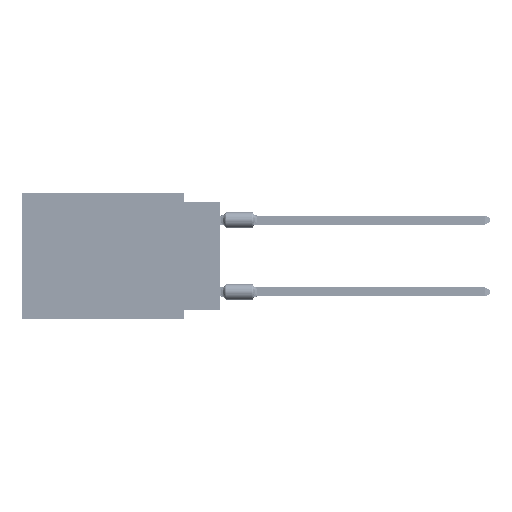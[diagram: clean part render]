
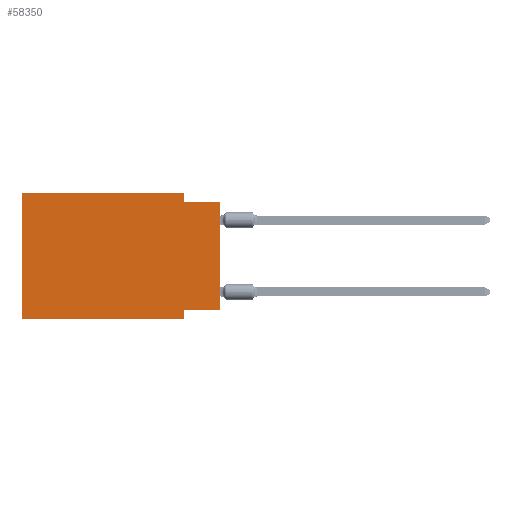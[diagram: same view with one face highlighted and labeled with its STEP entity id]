
A CAD part, left-side view. The second image highlights one B-rep face of the part: STEP entity #58350.
In plain terms, the highlighted planar face has unit normal (-1, 0, 0).
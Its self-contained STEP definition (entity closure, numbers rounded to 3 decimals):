
#297 = DIRECTION ( 'NONE',  ( 0., 0., -1. ) ) ;
#375 = EDGE_CURVE ( 'NONE', #9634, #56281, #20142, .T. ) ;
#571 = VECTOR ( 'NONE', #66476, 1000. ) ;
#1052 = EDGE_CURVE ( 'NONE', #13156, #18423, #66818, .T. ) ;
#1250 = CARTESIAN_POINT ( 'NONE',  ( 0., 0., -8.255 ) ) ;
#3083 = DIRECTION ( 'NONE',  ( 0., -1., 0. ) ) ;
#5361 = DIRECTION ( 'NONE',  ( 1., 0., 0. ) ) ;
#8237 = EDGE_CURVE ( 'NONE', #26276, #27778, #59389, .T. ) ;
#8367 = DIRECTION ( 'NONE',  ( 0., 0., -1. ) ) ;
#9634 = VERTEX_POINT ( 'NONE', #28352 ) ;
#13156 = VERTEX_POINT ( 'NONE', #1250 ) ;
#13600 = CARTESIAN_POINT ( 'NONE',  ( 0., 2.54, 0. ) ) ;
#13890 = DIRECTION ( 'NONE',  ( 0., 0., 1. ) ) ;
#17113 = LINE ( 'NONE', #42981, #43524 ) ;
#18196 = ORIENTED_EDGE ( 'NONE', *, *, #46962, .F. ) ;
#18423 = VERTEX_POINT ( 'NONE', #36624 ) ;
#19375 = DIRECTION ( 'NONE',  ( 0., 1., 0. ) ) ;
#19699 = LINE ( 'NONE', #50859, #60046 ) ;
#20142 = LINE ( 'NONE', #31317, #51988 ) ;
#20844 = ORIENTED_EDGE ( 'NONE', *, *, #36057, .F. ) ;
#22134 = FACE_OUTER_BOUND ( 'NONE', #61054, .T. ) ;
#22450 = CARTESIAN_POINT ( 'NONE',  ( 0., 2.54, 0. ) ) ;
#24410 = VERTEX_POINT ( 'NONE', #68176 ) ;
#25674 = CARTESIAN_POINT ( 'NONE',  ( 0., 2.54, -8.89 ) ) ;
#26276 = VERTEX_POINT ( 'NONE', #50204 ) ;
#27778 = VERTEX_POINT ( 'NONE', #25674 ) ;
#28079 = DIRECTION ( 'NONE',  ( 0., 0., -1. ) ) ;
#28352 = CARTESIAN_POINT ( 'NONE',  ( 0., 13.97, -8.89 ) ) ;
#29003 = VECTOR ( 'NONE', #67531, 1000. ) ;
#30300 = ORIENTED_EDGE ( 'NONE', *, *, #1052, .T. ) ;
#31317 = CARTESIAN_POINT ( 'NONE',  ( 0., 13.97, 0. ) ) ;
#33422 = ORIENTED_EDGE ( 'NONE', *, *, #44740, .F. ) ;
#34199 = LINE ( 'NONE', #62176, #40114 ) ;
#34949 = ORIENTED_EDGE ( 'NONE', *, *, #44660, .T. ) ;
#36057 = EDGE_CURVE ( 'NONE', #46064, #24410, #40180, .T. ) ;
#36302 = ORIENTED_EDGE ( 'NONE', *, *, #42102, .F. ) ;
#36624 = CARTESIAN_POINT ( 'NONE',  ( 0., 0., -0.635 ) ) ;
#37562 = ORIENTED_EDGE ( 'NONE', *, *, #375, .F. ) ;
#39874 = CARTESIAN_POINT ( 'NONE',  ( 0., 0., 0. ) ) ;
#40114 = VECTOR ( 'NONE', #3083, 1000. ) ;
#40180 = LINE ( 'NONE', #13600, #56267 ) ;
#42102 = EDGE_CURVE ( 'NONE', #56281, #46064, #34199, .T. ) ;
#42768 = CARTESIAN_POINT ( 'NONE',  ( 0., 13.97, 0. ) ) ;
#42971 = VECTOR ( 'NONE', #297, 1000. ) ;
#42981 = CARTESIAN_POINT ( 'NONE',  ( 0., 0., -0.635 ) ) ;
#43524 = VECTOR ( 'NONE', #59088, 1000. ) ;
#43825 = PLANE ( 'NONE',  #63961 ) ;
#44660 = EDGE_CURVE ( 'NONE', #9634, #27778, #68890, .T. ) ;
#44740 = EDGE_CURVE ( 'NONE', #24410, #18423, #17113, .T. ) ;
#46064 = VERTEX_POINT ( 'NONE', #22450 ) ;
#46856 = CARTESIAN_POINT ( 'NONE',  ( 0., 13.97, -8.89 ) ) ;
#46962 = EDGE_CURVE ( 'NONE', #13156, #26276, #19699, .T. ) ;
#50204 = CARTESIAN_POINT ( 'NONE',  ( 0., 2.54, -8.255 ) ) ;
#50859 = CARTESIAN_POINT ( 'NONE',  ( 0., 0., -8.255 ) ) ;
#51988 = VECTOR ( 'NONE', #13890, 1000. ) ;
#56267 = VECTOR ( 'NONE', #8367, 1000. ) ;
#56281 = VERTEX_POINT ( 'NONE', #58368 ) ;
#58350 = ADVANCED_FACE ( 'NONE', ( #22134 ), #43825, .F. ) ;
#58353 = CARTESIAN_POINT ( 'NONE',  ( 0., 2.54, -8.89 ) ) ;
#58368 = CARTESIAN_POINT ( 'NONE',  ( 0., 13.97, 0. ) ) ;
#59088 = DIRECTION ( 'NONE',  ( 0., -1., 0. ) ) ;
#59389 = LINE ( 'NONE', #58353, #42971 ) ;
#60046 = VECTOR ( 'NONE', #19375, 1000. ) ;
#61054 = EDGE_LOOP ( 'NONE', ( #30300, #33422, #20844, #36302, #37562, #34949, #62924, #18196 ) ) ;
#62176 = CARTESIAN_POINT ( 'NONE',  ( 0., 13.97, 0. ) ) ;
#62924 = ORIENTED_EDGE ( 'NONE', *, *, #8237, .F. ) ;
#63961 = AXIS2_PLACEMENT_3D ( 'NONE', #42768, #5361, #28079 ) ;
#66476 = DIRECTION ( 'NONE',  ( 0., 0., 1. ) ) ;
#66818 = LINE ( 'NONE', #39874, #571 ) ;
#67531 = DIRECTION ( 'NONE',  ( 0., -1., 0. ) ) ;
#68176 = CARTESIAN_POINT ( 'NONE',  ( 0., 2.54, -0.635 ) ) ;
#68890 = LINE ( 'NONE', #46856, #29003 ) ;
